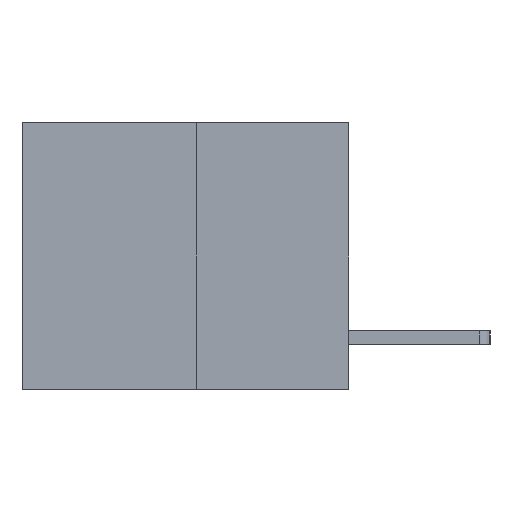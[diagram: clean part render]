
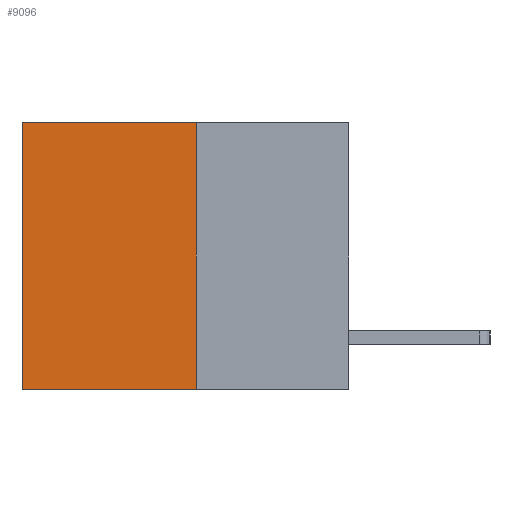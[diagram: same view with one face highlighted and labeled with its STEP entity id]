
A CAD part, left-side view. The second image highlights one B-rep face of the part: STEP entity #9096.
In plain terms, the highlighted planar face has unit normal (-1, 0, 0).
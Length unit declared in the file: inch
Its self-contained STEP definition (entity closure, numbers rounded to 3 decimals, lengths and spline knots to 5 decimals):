
#982 = LINE ( 'NONE', #3685, #9832 ) ;
#1000 = DIRECTION ( 'NONE',  ( 1., 0., 0. ) ) ;
#1913 = VECTOR ( 'NONE', #4768, 39.37008 ) ;
#1923 = VERTEX_POINT ( 'NONE', #9385 ) ;
#2432 = EDGE_CURVE ( 'NONE', #1923, #5826, #6789, .T. ) ;
#2498 = DIRECTION ( 'NONE',  ( 0., 0., -1. ) ) ;
#2752 = FACE_OUTER_BOUND ( 'NONE', #9664, .T. ) ;
#3376 = EDGE_CURVE ( 'NONE', #1923, #9009, #9569, .T. ) ;
#3685 = CARTESIAN_POINT ( 'NONE',  ( 0.3165, 0.6, -0.49 ) ) ;
#3792 = DIRECTION ( 'NONE',  ( 0., 0., -1. ) ) ;
#4091 = CARTESIAN_POINT ( 'NONE',  ( 0.3165, 0.28, -0.49 ) ) ;
#4129 = DIRECTION ( 'NONE',  ( 0., 1., 0. ) ) ;
#4321 = EDGE_CURVE ( 'NONE', #5826, #10887, #6592, .T. ) ;
#4645 = ORIENTED_EDGE ( 'NONE', *, *, #10624, .T. ) ;
#4768 = DIRECTION ( 'NONE',  ( 0., 1., 0. ) ) ;
#5185 = AXIS2_PLACEMENT_3D ( 'NONE', #8597, #1000, #9571 ) ;
#5826 = VERTEX_POINT ( 'NONE', #9068 ) ;
#6509 = VECTOR ( 'NONE', #2498, 39.37008 ) ;
#6592 = LINE ( 'NONE', #9149, #1913 ) ;
#6789 = LINE ( 'NONE', #4091, #6509 ) ;
#7583 = CARTESIAN_POINT ( 'NONE',  ( 0.3165, 0.28, 0. ) ) ;
#7781 = PLANE ( 'NONE',  #5185 ) ;
#8597 = CARTESIAN_POINT ( 'NONE',  ( 0.3165, 0.28, -0.49 ) ) ;
#8770 = ORIENTED_EDGE ( 'NONE', *, *, #3376, .T. ) ;
#9009 = VERTEX_POINT ( 'NONE', #11067 ) ;
#9068 = CARTESIAN_POINT ( 'NONE',  ( 0.3165, 0.28, -0.49 ) ) ;
#9096 = ADVANCED_FACE ( 'NONE', ( #2752 ), #7781, .F. ) ;
#9149 = CARTESIAN_POINT ( 'NONE',  ( 0.3165, 0.28, -0.49 ) ) ;
#9385 = CARTESIAN_POINT ( 'NONE',  ( 0.3165, 0.28, 0. ) ) ;
#9569 = LINE ( 'NONE', #7583, #10793 ) ;
#9571 = DIRECTION ( 'NONE',  ( 0., 0., -1. ) ) ;
#9664 = EDGE_LOOP ( 'NONE', ( #4645, #10339, #10651, #8770 ) ) ;
#9774 = CARTESIAN_POINT ( 'NONE',  ( 0.3165, 0.6, -0.49 ) ) ;
#9832 = VECTOR ( 'NONE', #3792, 39.37008 ) ;
#10339 = ORIENTED_EDGE ( 'NONE', *, *, #4321, .F. ) ;
#10624 = EDGE_CURVE ( 'NONE', #9009, #10887, #982, .T. ) ;
#10651 = ORIENTED_EDGE ( 'NONE', *, *, #2432, .F. ) ;
#10793 = VECTOR ( 'NONE', #4129, 39.37008 ) ;
#10887 = VERTEX_POINT ( 'NONE', #9774 ) ;
#11067 = CARTESIAN_POINT ( 'NONE',  ( 0.3165, 0.6, 0. ) ) ;
